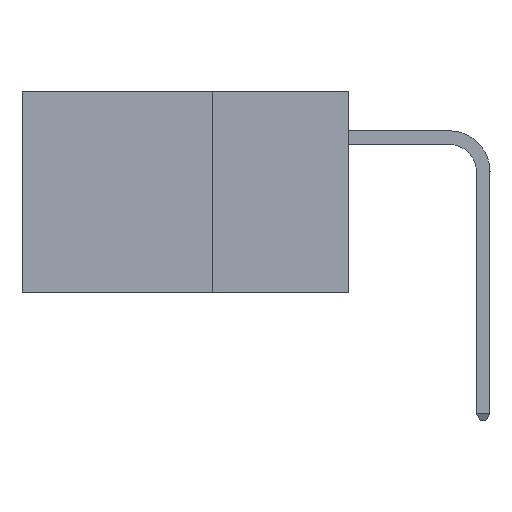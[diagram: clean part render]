
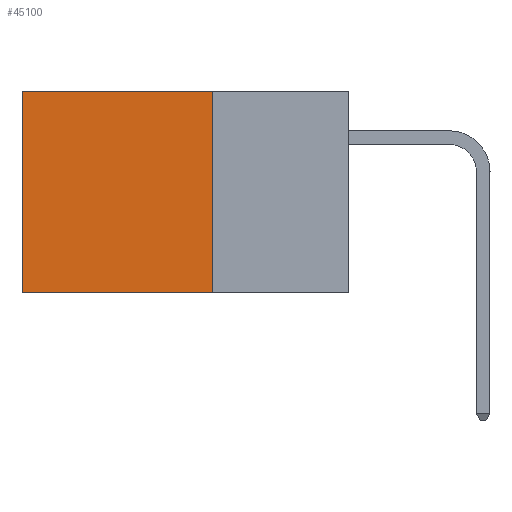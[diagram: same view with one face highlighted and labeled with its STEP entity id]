
A CAD part, left-side view. The second image highlights one B-rep face of the part: STEP entity #45100.
In plain terms, the highlighted planar face has unit normal (-1, 0, 0).
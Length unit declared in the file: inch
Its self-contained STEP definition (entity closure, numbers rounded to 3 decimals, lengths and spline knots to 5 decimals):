
#472 = CARTESIAN_POINT ( 'NONE',  ( 0.2875, 0.6, -0.37 ) ) ;
#1133 = VECTOR ( 'NONE', #20570, 39.37008 ) ;
#1765 = DIRECTION ( 'NONE',  ( 0., 1., 0. ) ) ;
#2393 = LINE ( 'NONE', #12858, #1133 ) ;
#2872 = CARTESIAN_POINT ( 'NONE',  ( 0.2875, 0.25, 0. ) ) ;
#5025 = VERTEX_POINT ( 'NONE', #49097 ) ;
#5464 = LINE ( 'NONE', #41961, #35561 ) ;
#6361 = AXIS2_PLACEMENT_3D ( 'NONE', #2872, #34346, #10862 ) ;
#8119 = CARTESIAN_POINT ( 'NONE',  ( 0.2875, 0.6, 0. ) ) ;
#8980 = ORIENTED_EDGE ( 'NONE', *, *, #22166, .T. ) ;
#10213 = FACE_OUTER_BOUND ( 'NONE', #11833, .T. ) ;
#10862 = DIRECTION ( 'NONE',  ( 0., 0., -1. ) ) ;
#11833 = EDGE_LOOP ( 'NONE', ( #38844, #15815, #32210, #8980 ) ) ;
#12078 = CARTESIAN_POINT ( 'NONE',  ( 0.2875, 0.25, 0. ) ) ;
#12858 = CARTESIAN_POINT ( 'NONE',  ( 0.2875, 0.25, -0.37 ) ) ;
#14780 = VERTEX_POINT ( 'NONE', #472 ) ;
#15240 = VERTEX_POINT ( 'NONE', #8119 ) ;
#15815 = ORIENTED_EDGE ( 'NONE', *, *, #36504, .F. ) ;
#19235 = LINE ( 'NONE', #30178, #20464 ) ;
#20464 = VECTOR ( 'NONE', #38312, 39.37008 ) ;
#20570 = DIRECTION ( 'NONE',  ( 0., 1., 0. ) ) ;
#22166 = EDGE_CURVE ( 'NONE', #35249, #15240, #41985, .T. ) ;
#26012 = EDGE_CURVE ( 'NONE', #15240, #14780, #5464, .T. ) ;
#30178 = CARTESIAN_POINT ( 'NONE',  ( 0.2875, 0.25, 0. ) ) ;
#30430 = PLANE ( 'NONE',  #6361 ) ;
#31608 = VECTOR ( 'NONE', #1765, 39.37008 ) ;
#32210 = ORIENTED_EDGE ( 'NONE', *, *, #34445, .F. ) ;
#34346 = DIRECTION ( 'NONE',  ( 1., 0., 0. ) ) ;
#34445 = EDGE_CURVE ( 'NONE', #35249, #5025, #19235, .T. ) ;
#35249 = VERTEX_POINT ( 'NONE', #12078 ) ;
#35561 = VECTOR ( 'NONE', #45841, 39.37008 ) ;
#36504 = EDGE_CURVE ( 'NONE', #5025, #14780, #2393, .T. ) ;
#37004 = CARTESIAN_POINT ( 'NONE',  ( 0.2875, 0.25, 0. ) ) ;
#38312 = DIRECTION ( 'NONE',  ( 0., 0., -1. ) ) ;
#38844 = ORIENTED_EDGE ( 'NONE', *, *, #26012, .T. ) ;
#41961 = CARTESIAN_POINT ( 'NONE',  ( 0.2875, 0.6, 0. ) ) ;
#41985 = LINE ( 'NONE', #37004, #31608 ) ;
#45100 = ADVANCED_FACE ( 'NONE', ( #10213 ), #30430, .F. ) ;
#45841 = DIRECTION ( 'NONE',  ( 0., 0., -1. ) ) ;
#49097 = CARTESIAN_POINT ( 'NONE',  ( 0.2875, 0.25, -0.37 ) ) ;
